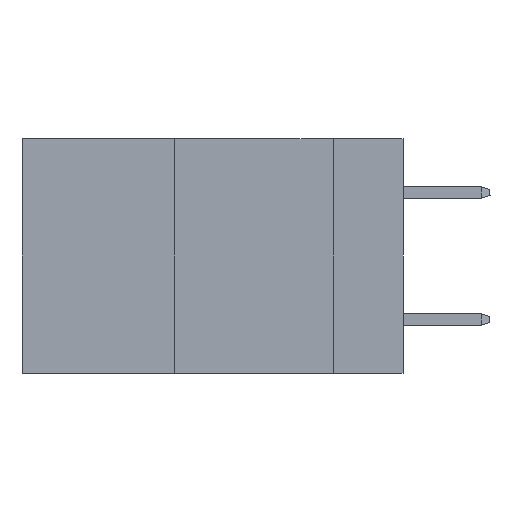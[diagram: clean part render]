
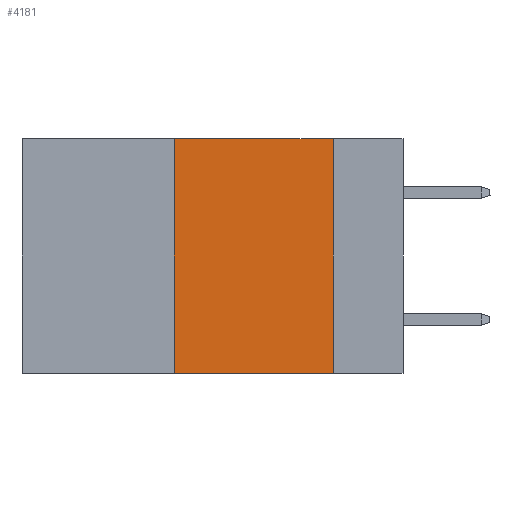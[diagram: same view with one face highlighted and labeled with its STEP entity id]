
A CAD part, left-side view. The second image highlights one B-rep face of the part: STEP entity #4181.
In plain terms, the highlighted planar face has unit normal (-1, 0, 0).
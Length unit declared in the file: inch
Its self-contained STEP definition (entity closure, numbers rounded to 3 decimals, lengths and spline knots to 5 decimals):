
#695 = DIRECTION ( 'NONE',  ( 0., 0., -1. ) ) ;
#2090 = DIRECTION ( 'NONE',  ( 0., -1., 0. ) ) ;
#2196 = VECTOR ( 'NONE', #695, 39.37008 ) ;
#2236 = CARTESIAN_POINT ( 'NONE',  ( 0., 0.36, 0. ) ) ;
#2260 = LINE ( 'NONE', #14908, #2196 ) ;
#3164 = VECTOR ( 'NONE', #9030, 39.37008 ) ;
#3479 = VERTEX_POINT ( 'NONE', #15871 ) ;
#4181 = ADVANCED_FACE ( 'NONE', ( #7233 ), #6049, .F. ) ;
#4901 = EDGE_CURVE ( 'NONE', #14477, #10953, #2260, .T. ) ;
#6049 = PLANE ( 'NONE',  #17725 ) ;
#6092 = DIRECTION ( 'NONE',  ( 0., 0., 1. ) ) ;
#6312 = ORIENTED_EDGE ( 'NONE', *, *, #4901, .F. ) ;
#6974 = VECTOR ( 'NONE', #2090, 39.37008 ) ;
#7233 = FACE_OUTER_BOUND ( 'NONE', #17671, .T. ) ;
#7261 = VERTEX_POINT ( 'NONE', #9515 ) ;
#7831 = LINE ( 'NONE', #14716, #3164 ) ;
#8733 = DIRECTION ( 'NONE',  ( 1., 0., 0. ) ) ;
#9030 = DIRECTION ( 'NONE',  ( 0., -1., 0. ) ) ;
#9515 = CARTESIAN_POINT ( 'NONE',  ( 0., 0.36, -0.37 ) ) ;
#10230 = CARTESIAN_POINT ( 'NONE',  ( 0., 0.11, 0. ) ) ;
#10234 = LINE ( 'NONE', #2236, #10321 ) ;
#10321 = VECTOR ( 'NONE', #6092, 39.37008 ) ;
#10411 = ORIENTED_EDGE ( 'NONE', *, *, #15320, .F. ) ;
#10466 = ORIENTED_EDGE ( 'NONE', *, *, #16474, .F. ) ;
#10514 = LINE ( 'NONE', #13460, #6974 ) ;
#10953 = VERTEX_POINT ( 'NONE', #12895 ) ;
#11946 = EDGE_CURVE ( 'NONE', #7261, #10953, #10514, .T. ) ;
#12895 = CARTESIAN_POINT ( 'NONE',  ( 0., 0.11, -0.37 ) ) ;
#13460 = CARTESIAN_POINT ( 'NONE',  ( 0., 0.6, -0.37 ) ) ;
#14477 = VERTEX_POINT ( 'NONE', #10230 ) ;
#14716 = CARTESIAN_POINT ( 'NONE',  ( 0., 0.6, 0. ) ) ;
#14908 = CARTESIAN_POINT ( 'NONE',  ( 0., 0.11, 0. ) ) ;
#15073 = ORIENTED_EDGE ( 'NONE', *, *, #11946, .T. ) ;
#15320 = EDGE_CURVE ( 'NONE', #7261, #3479, #10234, .T. ) ;
#15871 = CARTESIAN_POINT ( 'NONE',  ( 0., 0.36, 0. ) ) ;
#15897 = CARTESIAN_POINT ( 'NONE',  ( 0., 0.6, 0. ) ) ;
#16474 = EDGE_CURVE ( 'NONE', #3479, #14477, #7831, .T. ) ;
#17250 = DIRECTION ( 'NONE',  ( 0., 0., -1. ) ) ;
#17671 = EDGE_LOOP ( 'NONE', ( #6312, #10466, #10411, #15073 ) ) ;
#17725 = AXIS2_PLACEMENT_3D ( 'NONE', #15897, #8733, #17250 ) ;
